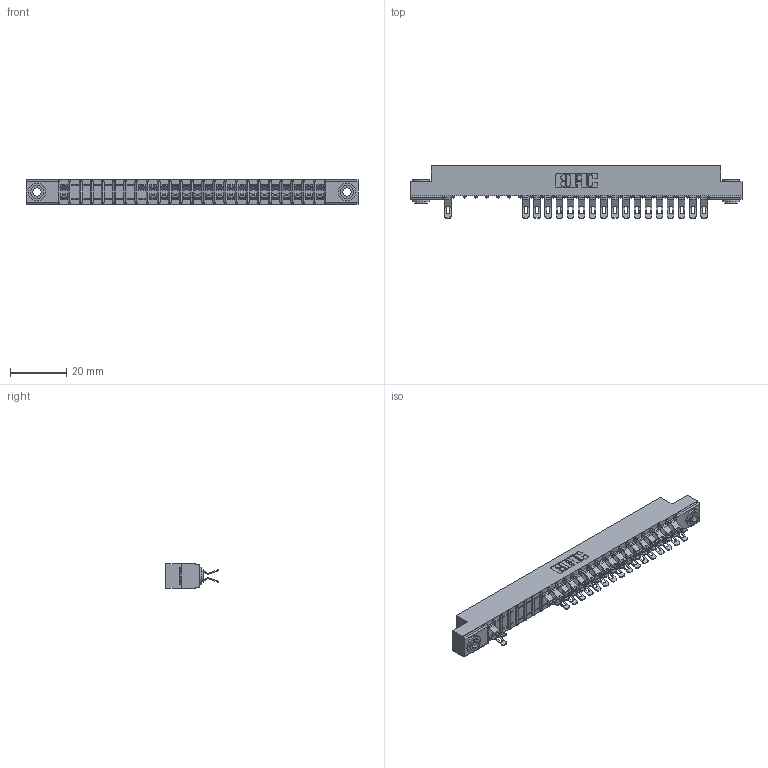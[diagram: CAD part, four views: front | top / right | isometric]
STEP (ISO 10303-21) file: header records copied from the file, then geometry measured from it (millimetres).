
FILE_DESCRIPTION (( 'STEP AP203' ), '1' );
FILE_NAME ('307-048-555-203.STEP', '2018-08-06T03:53:41', ( '' ), ( '' ), 'SwSTEP 2.0', 'SolidWorks 2016', '' );
FILE_SCHEMA (( 'CONFIG_CONTROL_DESIGN' ));
Length unit declared in the file: inch
Products named in the file (4): 345-250-002_345-250-002-102; 307-048-555-203; 307 Part_.156 Dia Mounting Holes; 307-290-001_555
Assembly tree (38 placements, depth 2):
  307-048-555-203
    307 Part_.156 Dia Mounting Holes
    307-290-001_555  x35
    345-250-002_345-250-002-102  x2
Bounding box: 118.11 x 18.75 x 8.71 mm (x, y, z)
Volume: 7662.7 mm3; surface area: 13467.7 mm2
Topology: 38 solids, 38 shells, 2460 faces, 7186 edges, 4672 vertices
Faces by surface type: plane 1362, cylinder 1040, sphere 50, cone 8
Entity records: 24748 total; most frequent: CARTESIAN_POINT 4096, ORIENTED_EDGE 4064, DIRECTION 4028, EDGE_CURVE 2032, VECTOR 1532, LINE 1532, VERTEX_POINT 1316, AXIS2_PLACEMENT_3D 1248
